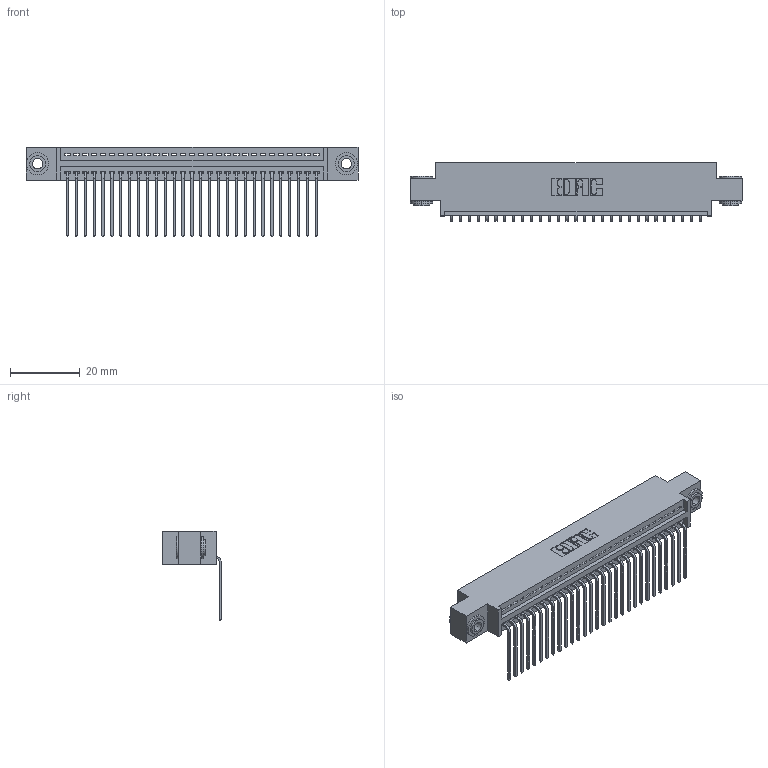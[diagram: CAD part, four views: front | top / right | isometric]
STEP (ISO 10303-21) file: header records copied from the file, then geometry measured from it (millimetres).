
FILE_DESCRIPTION (( 'STEP AP203' ), '1' );
FILE_NAME ('395-029-559-603.STEP', '2019-10-19T06:13:54', ( '' ), ( '' ), 'SwSTEP 2.0', 'SolidWorks 2016', '' );
FILE_SCHEMA (( 'CONFIG_CONTROL_DESIGN' ));
Length unit declared in the file: inch
Products named in the file (4): 345-292-001_558 559 Tail - 1; 395-029-559-603; 345 Part_0.170 Offset - 0.156 Dia-TH; 345-250-002_345-250-002-102
Assembly tree (32 placements, depth 2):
  395-029-559-603
    345 Part_0.170 Offset - 0.156 Dia-TH
    345-292-001_558 559 Tail - 1  x29
    345-250-002_345-250-002-102  x2
Bounding box: 94.87 x 16.75 x 25.53 mm (x, y, z)
Volume: 8906.9 mm3; surface area: 12568.6 mm2
Topology: 32 solids, 32 shells, 1908 faces, 5707 edges, 3762 vertices
Faces by surface type: plane 1312, cylinder 588, cone 8
Entity records: 24442 total; most frequent: CARTESIAN_POINT 4214, ORIENTED_EDGE 4170, DIRECTION 3729, EDGE_CURVE 2085, VECTOR 1813, LINE 1813, VERTEX_POINT 1386, AXIS2_PLACEMENT_3D 958
